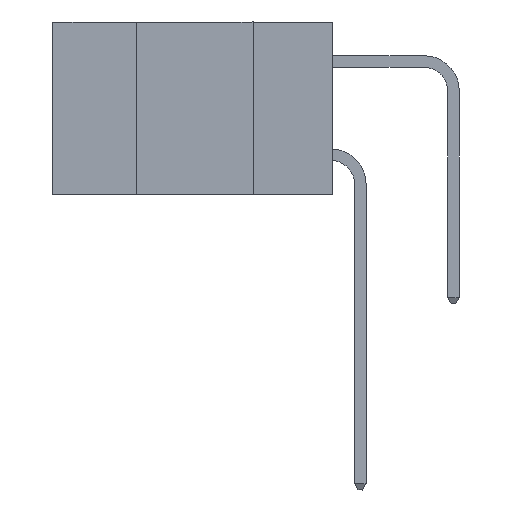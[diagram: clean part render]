
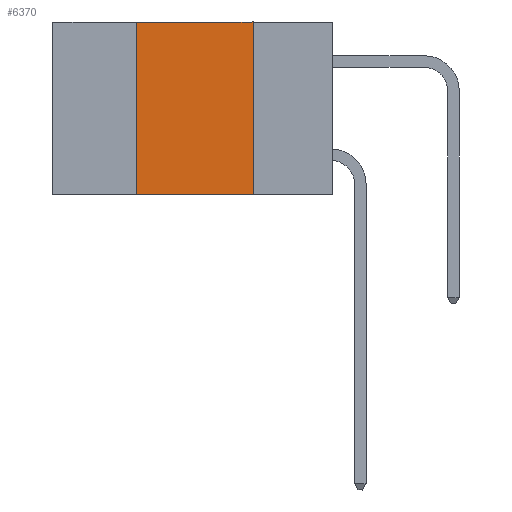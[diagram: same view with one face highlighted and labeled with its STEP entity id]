
A CAD part, left-side view. The second image highlights one B-rep face of the part: STEP entity #6370.
In plain terms, the highlighted planar face has unit normal (-1, 0, 0).
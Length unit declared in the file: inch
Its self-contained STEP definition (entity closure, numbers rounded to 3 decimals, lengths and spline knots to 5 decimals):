
#795 = EDGE_LOOP ( 'NONE', ( #10276, #6857, #11359, #13543 ) ) ;
#1011 = DIRECTION ( 'NONE',  ( 1., 0., 0. ) ) ;
#1273 = VERTEX_POINT ( 'NONE', #12228 ) ;
#1759 = LINE ( 'NONE', #10407, #6343 ) ;
#2295 = EDGE_CURVE ( 'NONE', #1273, #6046, #9108, .T. ) ;
#2693 = EDGE_CURVE ( 'NONE', #4528, #6046, #7666, .T. ) ;
#3493 = CARTESIAN_POINT ( 'NONE',  ( 0., 0.17, -0.37 ) ) ;
#3677 = CARTESIAN_POINT ( 'NONE',  ( 0., 0.6, 0. ) ) ;
#3749 = LINE ( 'NONE', #3677, #4776 ) ;
#3778 = DIRECTION ( 'NONE',  ( 0., 0., -1. ) ) ;
#4275 = CARTESIAN_POINT ( 'NONE',  ( 0., 0.6, 0. ) ) ;
#4528 = VERTEX_POINT ( 'NONE', #5361 ) ;
#4776 = VECTOR ( 'NONE', #9366, 39.37008 ) ;
#5361 = CARTESIAN_POINT ( 'NONE',  ( 0., 0.42, -0.37 ) ) ;
#5953 = DIRECTION ( 'NONE',  ( 0., 0., 1. ) ) ;
#6046 = VERTEX_POINT ( 'NONE', #3493 ) ;
#6085 = CARTESIAN_POINT ( 'NONE',  ( 0., 0.42, 0. ) ) ;
#6343 = VECTOR ( 'NONE', #5953, 39.37008 ) ;
#6370 = ADVANCED_FACE ( 'NONE', ( #14104 ), #8804, .F. ) ;
#6857 = ORIENTED_EDGE ( 'NONE', *, *, #12316, .F. ) ;
#7459 = CARTESIAN_POINT ( 'NONE',  ( 0., 0.6, -0.37 ) ) ;
#7666 = LINE ( 'NONE', #7459, #12515 ) ;
#7983 = VERTEX_POINT ( 'NONE', #6085 ) ;
#8804 = PLANE ( 'NONE',  #11704 ) ;
#9108 = LINE ( 'NONE', #11188, #13223 ) ;
#9366 = DIRECTION ( 'NONE',  ( 0., -1., 0. ) ) ;
#10276 = ORIENTED_EDGE ( 'NONE', *, *, #2295, .F. ) ;
#10407 = CARTESIAN_POINT ( 'NONE',  ( 0., 0.42, -0.37 ) ) ;
#10574 = EDGE_CURVE ( 'NONE', #4528, #7983, #1759, .T. ) ;
#11188 = CARTESIAN_POINT ( 'NONE',  ( 0., 0.17, -0.37 ) ) ;
#11359 = ORIENTED_EDGE ( 'NONE', *, *, #10574, .F. ) ;
#11704 = AXIS2_PLACEMENT_3D ( 'NONE', #4275, #1011, #13177 ) ;
#11819 = DIRECTION ( 'NONE',  ( 0., -1., 0. ) ) ;
#12228 = CARTESIAN_POINT ( 'NONE',  ( 0., 0.17, 0. ) ) ;
#12316 = EDGE_CURVE ( 'NONE', #7983, #1273, #3749, .T. ) ;
#12515 = VECTOR ( 'NONE', #11819, 39.37008 ) ;
#13177 = DIRECTION ( 'NONE',  ( 0., 0., -1. ) ) ;
#13223 = VECTOR ( 'NONE', #3778, 39.37008 ) ;
#13543 = ORIENTED_EDGE ( 'NONE', *, *, #2693, .T. ) ;
#14104 = FACE_OUTER_BOUND ( 'NONE', #795, .T. ) ;
